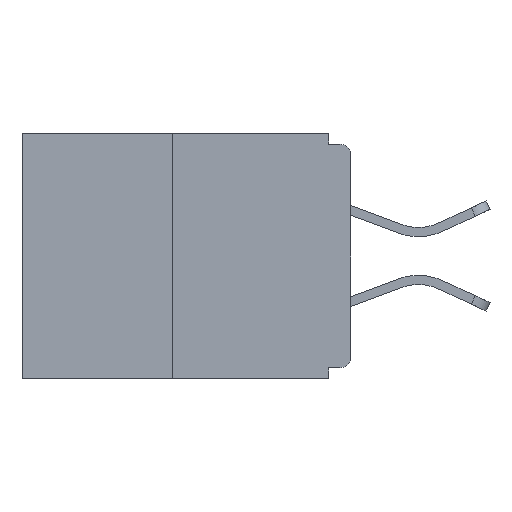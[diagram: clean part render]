
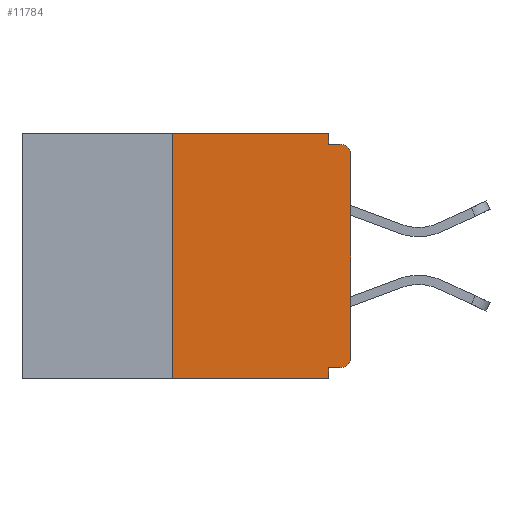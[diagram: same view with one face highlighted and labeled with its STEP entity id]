
A CAD part, left-side view. The second image highlights one B-rep face of the part: STEP entity #11784.
In plain terms, the highlighted planar face has unit normal (-1, 0, 0).
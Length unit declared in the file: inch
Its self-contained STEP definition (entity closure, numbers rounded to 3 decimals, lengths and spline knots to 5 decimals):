
#50 = CARTESIAN_POINT ( 'NONE',  ( 0., 0., -0.313 ) ) ;
#54 = CARTESIAN_POINT ( 'NONE',  ( 0., 0., -0.015 ) ) ;
#204 = DIRECTION ( 'NONE',  ( 0., -1., 0. ) ) ;
#229 = ORIENTED_EDGE ( 'NONE', *, *, #14066, .T. ) ;
#434 = FACE_OUTER_BOUND ( 'NONE', #1750, .T. ) ;
#497 = CARTESIAN_POINT ( 'NONE',  ( 0., 0., -0.03 ) ) ;
#951 = AXIS2_PLACEMENT_3D ( 'NONE', #6545, #991, #7706 ) ;
#991 = DIRECTION ( 'NONE',  ( -1., 0., 0. ) ) ;
#1334 = LINE ( 'NONE', #10231, #13634 ) ;
#1539 = DIRECTION ( 'NONE',  ( 0., -1., 0. ) ) ;
#1750 = EDGE_LOOP ( 'NONE', ( #2277, #3563, #10479, #2345, #13091, #3305, #13916, #229, #7067, #6486 ) ) ;
#1913 = VECTOR ( 'NONE', #7530, 39.37008 ) ;
#2277 = ORIENTED_EDGE ( 'NONE', *, *, #9899, .F. ) ;
#2299 = LINE ( 'NONE', #3469, #14223 ) ;
#2345 = ORIENTED_EDGE ( 'NONE', *, *, #2764, .F. ) ;
#2430 = LINE ( 'NONE', #9826, #2959 ) ;
#2545 = DIRECTION ( 'NONE',  ( 1., 0., 0. ) ) ;
#2613 = CARTESIAN_POINT ( 'NONE',  ( 0., 0.031, -0.328 ) ) ;
#2695 = EDGE_CURVE ( 'NONE', #3314, #8296, #2905, .T. ) ;
#2764 = EDGE_CURVE ( 'NONE', #10408, #8296, #2430, .T. ) ;
#2905 = LINE ( 'NONE', #7567, #5991 ) ;
#2941 = VERTEX_POINT ( 'NONE', #4978 ) ;
#2959 = VECTOR ( 'NONE', #5864, 39.37008 ) ;
#3006 = AXIS2_PLACEMENT_3D ( 'NONE', #9481, #8165, #5095 ) ;
#3151 = VERTEX_POINT ( 'NONE', #5492 ) ;
#3305 = ORIENTED_EDGE ( 'NONE', *, *, #6969, .T. ) ;
#3314 = VERTEX_POINT ( 'NONE', #5635 ) ;
#3469 = CARTESIAN_POINT ( 'NONE',  ( 0., 0.031, 0. ) ) ;
#3472 = DIRECTION ( 'NONE',  ( 0., 0., 1. ) ) ;
#3563 = ORIENTED_EDGE ( 'NONE', *, *, #9311, .F. ) ;
#4315 = LINE ( 'NONE', #13132, #1913 ) ;
#4978 = CARTESIAN_POINT ( 'NONE',  ( 0., 0.031, -0.015 ) ) ;
#5095 = DIRECTION ( 'NONE',  ( 0., 0., -1. ) ) ;
#5228 = EDGE_CURVE ( 'NONE', #8951, #6945, #9707, .T. ) ;
#5492 = CARTESIAN_POINT ( 'NONE',  ( 0., 0.015, -0.328 ) ) ;
#5635 = CARTESIAN_POINT ( 'NONE',  ( 0., 0.25, -0.343 ) ) ;
#5864 = DIRECTION ( 'NONE',  ( 0., 0., -1. ) ) ;
#5912 = DIRECTION ( 'NONE',  ( 0., 0., -1. ) ) ;
#5991 = VECTOR ( 'NONE', #13979, 39.37008 ) ;
#6486 = ORIENTED_EDGE ( 'NONE', *, *, #14157, .F. ) ;
#6502 = VECTOR ( 'NONE', #204, 39.37008 ) ;
#6545 = CARTESIAN_POINT ( 'NONE',  ( 0., 0.015, -0.03 ) ) ;
#6891 = LINE ( 'NONE', #10105, #11993 ) ;
#6945 = VERTEX_POINT ( 'NONE', #497 ) ;
#6969 = EDGE_CURVE ( 'NONE', #3151, #8951, #12074, .T. ) ;
#7067 = ORIENTED_EDGE ( 'NONE', *, *, #7292, .F. ) ;
#7292 = EDGE_CURVE ( 'NONE', #2941, #11947, #13405, .T. ) ;
#7511 = CARTESIAN_POINT ( 'NONE',  ( 0., 0.015, -0.015 ) ) ;
#7530 = DIRECTION ( 'NONE',  ( 0., 1., 0. ) ) ;
#7567 = CARTESIAN_POINT ( 'NONE',  ( 0., 0.46, -0.343 ) ) ;
#7602 = AXIS2_PLACEMENT_3D ( 'NONE', #9265, #2545, #5912 ) ;
#7604 = CARTESIAN_POINT ( 'NONE',  ( 0., 0.25, 0. ) ) ;
#7706 = DIRECTION ( 'NONE',  ( 0., 0., -1. ) ) ;
#7891 = VERTEX_POINT ( 'NONE', #7604 ) ;
#7935 = EDGE_CURVE ( 'NONE', #3151, #10408, #4315, .T. ) ;
#8165 = DIRECTION ( 'NONE',  ( -1., 0., 0. ) ) ;
#8296 = VERTEX_POINT ( 'NONE', #11842 ) ;
#8544 = DIRECTION ( 'NONE',  ( 0., 0., 1. ) ) ;
#8951 = VERTEX_POINT ( 'NONE', #50 ) ;
#9026 = DIRECTION ( 'NONE',  ( 0., 0., -1. ) ) ;
#9265 = CARTESIAN_POINT ( 'NONE',  ( 0., 0.46, 0. ) ) ;
#9311 = EDGE_CURVE ( 'NONE', #3314, #7891, #6891, .T. ) ;
#9481 = CARTESIAN_POINT ( 'NONE',  ( 0., 0.015, -0.313 ) ) ;
#9707 = LINE ( 'NONE', #10717, #13214 ) ;
#9826 = CARTESIAN_POINT ( 'NONE',  ( 0., 0.031, -0.343 ) ) ;
#9881 = VERTEX_POINT ( 'NONE', #12547 ) ;
#9899 = EDGE_CURVE ( 'NONE', #7891, #9881, #1334, .T. ) ;
#10105 = CARTESIAN_POINT ( 'NONE',  ( 0., 0.25, 0. ) ) ;
#10231 = CARTESIAN_POINT ( 'NONE',  ( 0., 0.46, 0. ) ) ;
#10256 = CIRCLE ( 'NONE', #951, 0.015 ) ;
#10408 = VERTEX_POINT ( 'NONE', #2613 ) ;
#10479 = ORIENTED_EDGE ( 'NONE', *, *, #2695, .T. ) ;
#10717 = CARTESIAN_POINT ( 'NONE',  ( 0., 0., 0. ) ) ;
#11784 = ADVANCED_FACE ( 'NONE', ( #434 ), #12531, .F. ) ;
#11842 = CARTESIAN_POINT ( 'NONE',  ( 0., 0.031, -0.343 ) ) ;
#11947 = VERTEX_POINT ( 'NONE', #7511 ) ;
#11993 = VECTOR ( 'NONE', #3472, 39.37008 ) ;
#12074 = CIRCLE ( 'NONE', #3006, 0.015 ) ;
#12531 = PLANE ( 'NONE',  #7602 ) ;
#12547 = CARTESIAN_POINT ( 'NONE',  ( 0., 0.031, 0. ) ) ;
#13091 = ORIENTED_EDGE ( 'NONE', *, *, #7935, .F. ) ;
#13132 = CARTESIAN_POINT ( 'NONE',  ( 0., 0., -0.328 ) ) ;
#13214 = VECTOR ( 'NONE', #8544, 39.37008 ) ;
#13405 = LINE ( 'NONE', #54, #6502 ) ;
#13634 = VECTOR ( 'NONE', #1539, 39.37008 ) ;
#13916 = ORIENTED_EDGE ( 'NONE', *, *, #5228, .T. ) ;
#13979 = DIRECTION ( 'NONE',  ( 0., -1., 0. ) ) ;
#14066 = EDGE_CURVE ( 'NONE', #6945, #11947, #10256, .T. ) ;
#14157 = EDGE_CURVE ( 'NONE', #9881, #2941, #2299, .T. ) ;
#14223 = VECTOR ( 'NONE', #9026, 39.37008 ) ;
